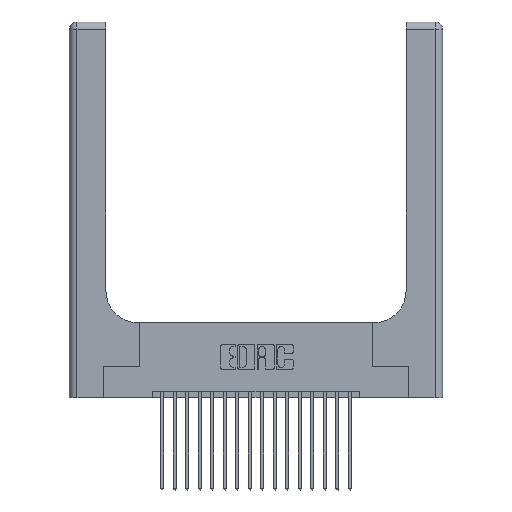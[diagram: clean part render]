
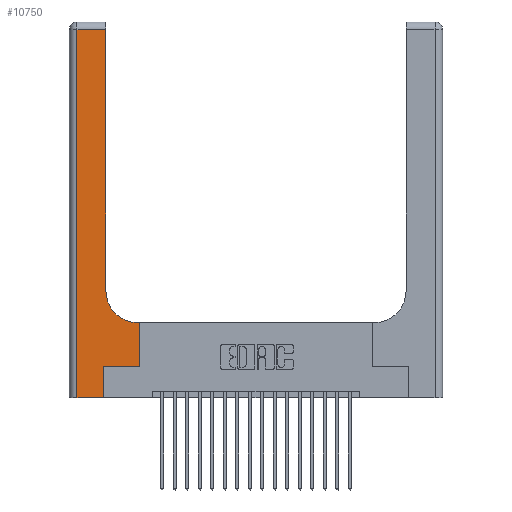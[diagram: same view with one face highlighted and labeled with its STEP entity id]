
A CAD part, top view. The second image highlights one B-rep face of the part: STEP entity #10750.
In plain terms, the highlighted planar face has unit normal (0, 0, 1).
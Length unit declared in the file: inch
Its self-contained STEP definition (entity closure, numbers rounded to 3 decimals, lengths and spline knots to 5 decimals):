
#205 = DIRECTION ( 'NONE',  ( 0., 0., -1. ) ) ;
#275 = CARTESIAN_POINT ( 'NONE',  ( 0.5415, 0.85, 0.37 ) ) ;
#733 = DIRECTION ( 'NONE',  ( -1., 0., 0. ) ) ;
#1192 = LINE ( 'NONE', #5380, #5187 ) ;
#1450 = CARTESIAN_POINT ( 'NONE',  ( 0.5585, 0.6, 0.37 ) ) ;
#2023 = DIRECTION ( 'NONE',  ( 1., 0., 0. ) ) ;
#2099 = CARTESIAN_POINT ( 'NONE',  ( 0.269, 0.25, 0.37 ) ) ;
#2929 = ORIENTED_EDGE ( 'NONE', *, *, #2982, .T. ) ;
#2982 = EDGE_CURVE ( 'NONE', #12597, #5398, #6456, .T. ) ;
#3198 = CARTESIAN_POINT ( 'NONE',  ( 0.06, 3., 0.37 ) ) ;
#3672 = CARTESIAN_POINT ( 'NONE',  ( 0.06, 2.94, 0.37 ) ) ;
#4341 = DIRECTION ( 'NONE',  ( 0., 1., 0. ) ) ;
#4446 = DIRECTION ( 'NONE',  ( -1., 0., 0. ) ) ;
#4624 = CARTESIAN_POINT ( 'NONE',  ( 0.269, 0., 0.37 ) ) ;
#4647 = CARTESIAN_POINT ( 'NONE',  ( 0.2915, 0.85, 0.37 ) ) ;
#4732 = VERTEX_POINT ( 'NONE', #4624 ) ;
#4735 = VERTEX_POINT ( 'NONE', #6286 ) ;
#4869 = DIRECTION ( 'NONE',  ( 0., -1., 0. ) ) ;
#5072 = VECTOR ( 'NONE', #733, 39.37008 ) ;
#5187 = VECTOR ( 'NONE', #7041, 39.37008 ) ;
#5380 = CARTESIAN_POINT ( 'NONE',  ( 0.269, 0.25, 0.37 ) ) ;
#5398 = VERTEX_POINT ( 'NONE', #1450 ) ;
#5782 = DIRECTION ( 'NONE',  ( 0., 1., 0. ) ) ;
#6023 = DIRECTION ( 'NONE',  ( 1., 0., 0. ) ) ;
#6286 = CARTESIAN_POINT ( 'NONE',  ( 0.06, 0., 0.37 ) ) ;
#6303 = LINE ( 'NONE', #14056, #18154 ) ;
#6456 = LINE ( 'NONE', #21118, #14503 ) ;
#6485 = ORIENTED_EDGE ( 'NONE', *, *, #16840, .T. ) ;
#6982 = VECTOR ( 'NONE', #4341, 39.37008 ) ;
#7041 = DIRECTION ( 'NONE',  ( 1., 0., 0. ) ) ;
#7953 = EDGE_CURVE ( 'NONE', #9513, #12597, #1192, .T. ) ;
#8412 = AXIS2_PLACEMENT_3D ( 'NONE', #275, #11890, #2023 ) ;
#8486 = VERTEX_POINT ( 'NONE', #21199 ) ;
#8656 = ORIENTED_EDGE ( 'NONE', *, *, #15744, .T. ) ;
#8756 = EDGE_CURVE ( 'NONE', #4732, #9513, #11775, .T. ) ;
#8811 = ORIENTED_EDGE ( 'NONE', *, *, #13437, .T. ) ;
#9010 = VERTEX_POINT ( 'NONE', #10025 ) ;
#9073 = CARTESIAN_POINT ( 'NONE',  ( 0., 2.94, 0.37 ) ) ;
#9513 = VERTEX_POINT ( 'NONE', #2099 ) ;
#10021 = ORIENTED_EDGE ( 'NONE', *, *, #7953, .T. ) ;
#10025 = CARTESIAN_POINT ( 'NONE',  ( 0.2915, 2.94, 0.37 ) ) ;
#10076 = CARTESIAN_POINT ( 'NONE',  ( 0., 3., 0.37 ) ) ;
#10750 = ADVANCED_FACE ( 'NONE', ( #13439 ), #19871, .F. ) ;
#10938 = CARTESIAN_POINT ( 'NONE',  ( 0.2915, 0.6, 0.37 ) ) ;
#11456 = EDGE_CURVE ( 'NONE', #9010, #17900, #13655, .T. ) ;
#11730 = EDGE_CURVE ( 'NONE', #17900, #4735, #12408, .T. ) ;
#11775 = LINE ( 'NONE', #12432, #6982 ) ;
#11804 = LINE ( 'NONE', #10938, #15589 ) ;
#11832 = DIRECTION ( 'NONE',  ( -1., 0., 0. ) ) ;
#11890 = DIRECTION ( 'NONE',  ( 0., 0., -1. ) ) ;
#12408 = LINE ( 'NONE', #3198, #20487 ) ;
#12432 = CARTESIAN_POINT ( 'NONE',  ( 0.269, 0., 0.37 ) ) ;
#12597 = VERTEX_POINT ( 'NONE', #14201 ) ;
#12636 = ORIENTED_EDGE ( 'NONE', *, *, #15537, .T. ) ;
#13314 = VECTOR ( 'NONE', #5782, 39.37008 ) ;
#13437 = EDGE_CURVE ( 'NONE', #15884, #9010, #17623, .T. ) ;
#13439 = FACE_OUTER_BOUND ( 'NONE', #18477, .T. ) ;
#13606 = CIRCLE ( 'NONE', #8412, 0.25 ) ;
#13655 = LINE ( 'NONE', #9073, #5072 ) ;
#13817 = CARTESIAN_POINT ( 'NONE',  ( 0.2915, 3., 0.37 ) ) ;
#14056 = CARTESIAN_POINT ( 'NONE',  ( 0., 0., 0.37 ) ) ;
#14201 = CARTESIAN_POINT ( 'NONE',  ( 0.5585, 0.25, 0.37 ) ) ;
#14503 = VECTOR ( 'NONE', #21050, 39.37008 ) ;
#15537 = EDGE_CURVE ( 'NONE', #8486, #15884, #13606, .T. ) ;
#15589 = VECTOR ( 'NONE', #4446, 39.37008 ) ;
#15744 = EDGE_CURVE ( 'NONE', #4735, #4732, #6303, .T. ) ;
#15884 = VERTEX_POINT ( 'NONE', #4647 ) ;
#16367 = ORIENTED_EDGE ( 'NONE', *, *, #11456, .T. ) ;
#16840 = EDGE_CURVE ( 'NONE', #5398, #8486, #11804, .T. ) ;
#17623 = LINE ( 'NONE', #13817, #13314 ) ;
#17900 = VERTEX_POINT ( 'NONE', #3672 ) ;
#18154 = VECTOR ( 'NONE', #6023, 39.37008 ) ;
#18343 = AXIS2_PLACEMENT_3D ( 'NONE', #10076, #205, #11832 ) ;
#18372 = ORIENTED_EDGE ( 'NONE', *, *, #11730, .T. ) ;
#18477 = EDGE_LOOP ( 'NONE', ( #8811, #16367, #18372, #8656, #20780, #10021, #2929, #6485, #12636 ) ) ;
#19871 = PLANE ( 'NONE',  #18343 ) ;
#20487 = VECTOR ( 'NONE', #4869, 39.37008 ) ;
#20780 = ORIENTED_EDGE ( 'NONE', *, *, #8756, .T. ) ;
#21050 = DIRECTION ( 'NONE',  ( 0., 1., 0. ) ) ;
#21118 = CARTESIAN_POINT ( 'NONE',  ( 0.5585, 0.25, 0.37 ) ) ;
#21199 = CARTESIAN_POINT ( 'NONE',  ( 0.5415, 0.6, 0.37 ) ) ;
